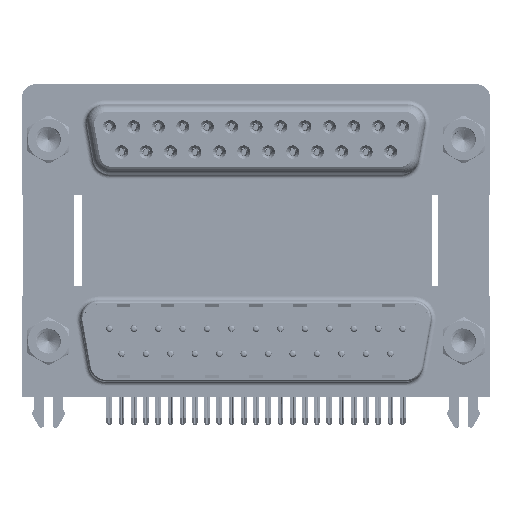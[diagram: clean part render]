
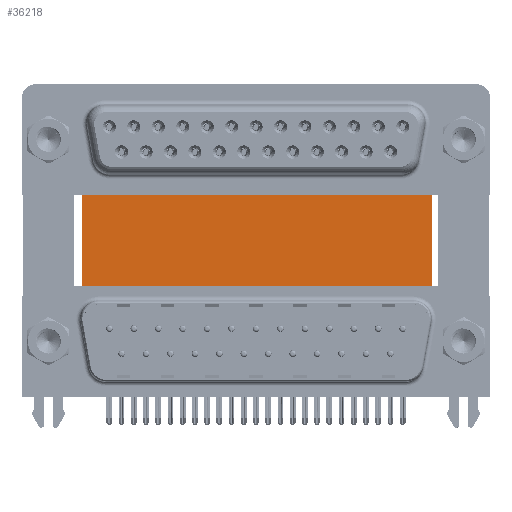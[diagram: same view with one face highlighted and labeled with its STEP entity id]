
A CAD part, top view. The second image highlights one B-rep face of the part: STEP entity #36218.
In plain terms, the highlighted planar face has unit normal (0, 0, 1).
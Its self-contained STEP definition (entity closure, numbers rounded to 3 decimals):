
#1199 = VECTOR ( 'NONE', #48315, 1000. ) ;
#2522 = LINE ( 'NONE', #35358, #8135 ) ;
#5676 = CARTESIAN_POINT ( 'NONE',  ( 43.43, 16.585, -12. ) ) ;
#6123 = DIRECTION ( 'NONE',  ( -1., 0., 0. ) ) ;
#8135 = VECTOR ( 'NONE', #26518, 1000. ) ;
#11464 = FACE_OUTER_BOUND ( 'NONE', #51658, .T. ) ;
#17993 = VERTEX_POINT ( 'NONE', #46462 ) ;
#20586 = VERTEX_POINT ( 'NONE', #38807 ) ;
#20640 = PLANE ( 'NONE',  #27138 ) ;
#26319 = ORIENTED_EDGE ( 'NONE', *, *, #47563, .F. ) ;
#26333 = VERTEX_POINT ( 'NONE', #39108 ) ;
#26369 = VERTEX_POINT ( 'NONE', #5676 ) ;
#26518 = DIRECTION ( 'NONE',  ( 0., -1., 0. ) ) ;
#27138 = AXIS2_PLACEMENT_3D ( 'NONE', #49015, #54707, #6123 ) ;
#29087 = CARTESIAN_POINT ( 'NONE',  ( 3.79, -3.735, -12. ) ) ;
#30366 = VECTOR ( 'NONE', #54049, 1000. ) ;
#34209 = DIRECTION ( 'NONE',  ( 0., -1., 0. ) ) ;
#34831 = CARTESIAN_POINT ( 'NONE',  ( 43.43, 16.585, -12. ) ) ;
#35358 = CARTESIAN_POINT ( 'NONE',  ( 3.79, 16.585, -12. ) ) ;
#36218 = ADVANCED_FACE ( 'NONE', ( #11464 ), #20640, .F. ) ;
#38807 = CARTESIAN_POINT ( 'NONE',  ( 3.79, 16.585, -12. ) ) ;
#39108 = CARTESIAN_POINT ( 'NONE',  ( 3.79, -3.735, -12. ) ) ;
#39555 = LINE ( 'NONE', #34831, #39907 ) ;
#39907 = VECTOR ( 'NONE', #34209, 1000. ) ;
#41494 = EDGE_CURVE ( 'NONE', #26333, #17993, #53050, .T. ) ;
#45717 = ORIENTED_EDGE ( 'NONE', *, *, #49382, .T. ) ;
#46462 = CARTESIAN_POINT ( 'NONE',  ( 43.43, -3.735, -12. ) ) ;
#47563 = EDGE_CURVE ( 'NONE', #20586, #26369, #53751, .T. ) ;
#48315 = DIRECTION ( 'NONE',  ( 1., 0., 0. ) ) ;
#49015 = CARTESIAN_POINT ( 'NONE',  ( 3.79, 16.585, -12. ) ) ;
#49382 = EDGE_CURVE ( 'NONE', #20586, #26333, #2522, .T. ) ;
#51658 = EDGE_LOOP ( 'NONE', ( #57926, #58106, #26319, #45717 ) ) ;
#53050 = LINE ( 'NONE', #29087, #1199 ) ;
#53751 = LINE ( 'NONE', #58768, #30366 ) ;
#54049 = DIRECTION ( 'NONE',  ( 1., 0., 0. ) ) ;
#54707 = DIRECTION ( 'NONE',  ( 0., 0., -1. ) ) ;
#57926 = ORIENTED_EDGE ( 'NONE', *, *, #41494, .T. ) ;
#58106 = ORIENTED_EDGE ( 'NONE', *, *, #58364, .F. ) ;
#58364 = EDGE_CURVE ( 'NONE', #26369, #17993, #39555, .T. ) ;
#58768 = CARTESIAN_POINT ( 'NONE',  ( 3.79, 16.585, -12. ) ) ;
